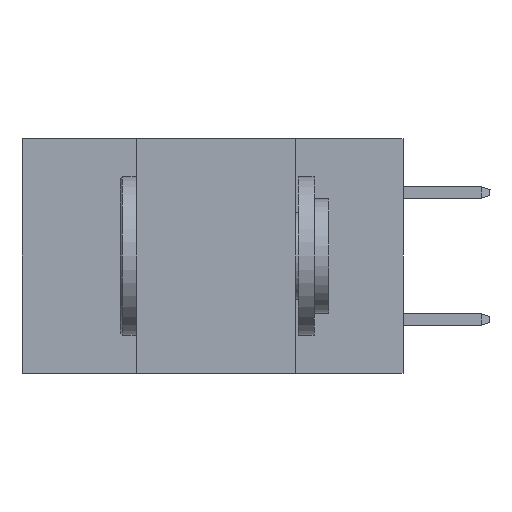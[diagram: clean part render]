
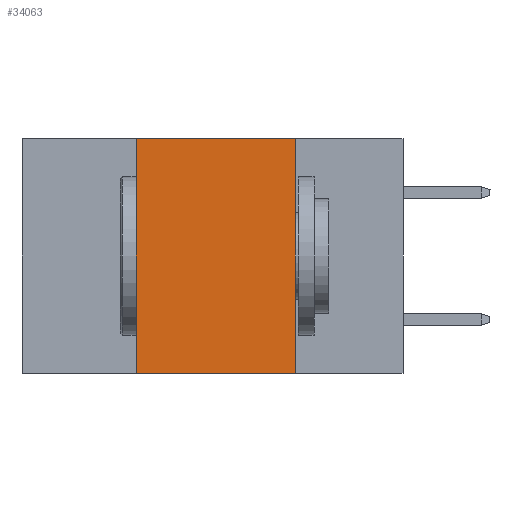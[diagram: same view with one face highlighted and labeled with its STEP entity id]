
A CAD part, left-side view. The second image highlights one B-rep face of the part: STEP entity #34063.
In plain terms, the highlighted planar face has unit normal (-1, 0, 0).
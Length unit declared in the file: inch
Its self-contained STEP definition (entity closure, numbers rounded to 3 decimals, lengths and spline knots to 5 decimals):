
#262 = CARTESIAN_POINT ( 'NONE',  ( 0., 0.42, -0.37 ) ) ;
#483 = VERTEX_POINT ( 'NONE', #14508 ) ;
#730 = EDGE_LOOP ( 'NONE', ( #32293, #29324, #29471, #1721 ) ) ;
#1523 = FACE_OUTER_BOUND ( 'NONE', #730, .T. ) ;
#1721 = ORIENTED_EDGE ( 'NONE', *, *, #25134, .T. ) ;
#5003 = CARTESIAN_POINT ( 'NONE',  ( 0., 0.6, 0. ) ) ;
#7154 = AXIS2_PLACEMENT_3D ( 'NONE', #5003, #18251, #15004 ) ;
#7500 = VECTOR ( 'NONE', #23334, 39.37008 ) ;
#8047 = CARTESIAN_POINT ( 'NONE',  ( 0., 0.17, 0. ) ) ;
#8146 = LINE ( 'NONE', #28395, #9496 ) ;
#9496 = VECTOR ( 'NONE', #38346, 39.37008 ) ;
#11773 = EDGE_CURVE ( 'NONE', #19746, #483, #26598, .T. ) ;
#14084 = CARTESIAN_POINT ( 'NONE',  ( 0., 0.6, 0. ) ) ;
#14508 = CARTESIAN_POINT ( 'NONE',  ( 0., 0.17, -0.37 ) ) ;
#15004 = DIRECTION ( 'NONE',  ( 0., 0., -1. ) ) ;
#17046 = VECTOR ( 'NONE', #39912, 39.37008 ) ;
#18228 = EDGE_CURVE ( 'NONE', #20729, #19746, #40207, .T. ) ;
#18251 = DIRECTION ( 'NONE',  ( 1., 0., 0. ) ) ;
#19205 = CARTESIAN_POINT ( 'NONE',  ( 0., 0.42, 0. ) ) ;
#19746 = VERTEX_POINT ( 'NONE', #8047 ) ;
#20317 = LINE ( 'NONE', #33603, #17046 ) ;
#20729 = VERTEX_POINT ( 'NONE', #19205 ) ;
#23334 = DIRECTION ( 'NONE',  ( 0., 0., -1. ) ) ;
#24791 = PLANE ( 'NONE',  #7154 ) ;
#25134 = EDGE_CURVE ( 'NONE', #33899, #483, #20317, .T. ) ;
#26598 = LINE ( 'NONE', #39848, #7500 ) ;
#28395 = CARTESIAN_POINT ( 'NONE',  ( 0., 0.42, 0. ) ) ;
#29324 = ORIENTED_EDGE ( 'NONE', *, *, #18228, .F. ) ;
#29471 = ORIENTED_EDGE ( 'NONE', *, *, #39671, .F. ) ;
#32293 = ORIENTED_EDGE ( 'NONE', *, *, #11773, .F. ) ;
#33603 = CARTESIAN_POINT ( 'NONE',  ( 0., 0.6, -0.37 ) ) ;
#33899 = VERTEX_POINT ( 'NONE', #262 ) ;
#34063 = ADVANCED_FACE ( 'NONE', ( #1523 ), #24791, .F. ) ;
#36921 = DIRECTION ( 'NONE',  ( 0., -1., 0. ) ) ;
#37062 = VECTOR ( 'NONE', #36921, 39.37008 ) ;
#38346 = DIRECTION ( 'NONE',  ( 0., 0., 1. ) ) ;
#39671 = EDGE_CURVE ( 'NONE', #33899, #20729, #8146, .T. ) ;
#39848 = CARTESIAN_POINT ( 'NONE',  ( 0., 0.17, 0. ) ) ;
#39912 = DIRECTION ( 'NONE',  ( 0., -1., 0. ) ) ;
#40207 = LINE ( 'NONE', #14084, #37062 ) ;
